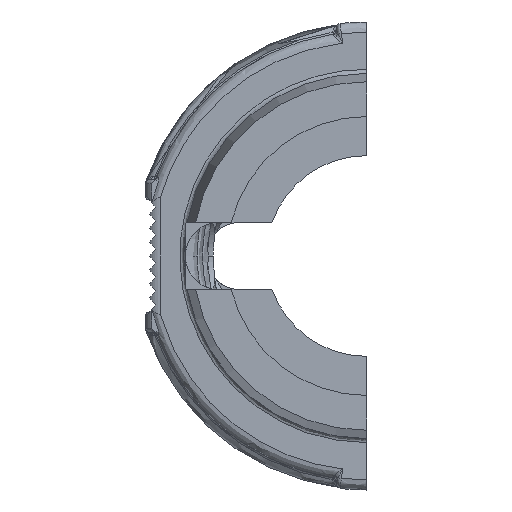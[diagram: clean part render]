
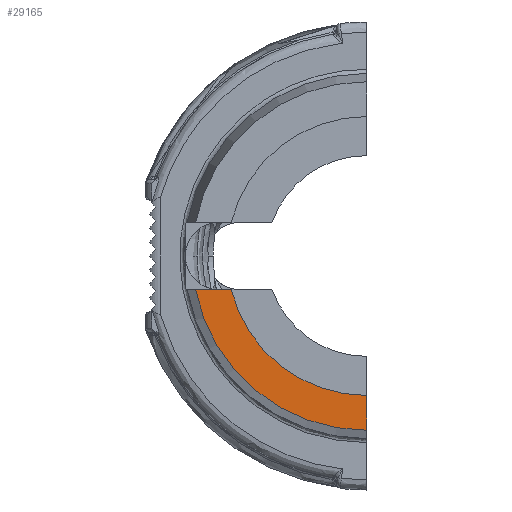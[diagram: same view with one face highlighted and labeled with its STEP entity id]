
A CAD part, left-side view. The second image highlights one B-rep face of the part: STEP entity #29165.
In plain terms, the highlighted planar face has unit normal (-1, 0, 0).
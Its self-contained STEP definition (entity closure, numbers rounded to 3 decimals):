
#5806 = DIRECTION ( 'NONE',  ( -1., 0., 0. ) ) ;
#8012 = AXIS2_PLACEMENT_3D ( 'NONE', #43436, #5806, #49741 ) ;
#8236 = CIRCLE ( 'NONE', #73202, 17.399 ) ;
#11814 = DIRECTION ( 'NONE',  ( 0., 1., 0. ) ) ;
#12703 = CARTESIAN_POINT ( 'NONE',  ( 0., 0., 0. ) ) ;
#12871 = CARTESIAN_POINT ( 'NONE',  ( 0., 0., 19.57 ) ) ;
#14411 = VECTOR ( 'NONE', #24136, 1000. ) ;
#19050 = DIRECTION ( 'NONE',  ( 0., -1., 0. ) ) ;
#19206 = DIRECTION ( 'NONE',  ( -1., 0., 0. ) ) ;
#22582 = VERTEX_POINT ( 'NONE', #62222 ) ;
#23591 = CARTESIAN_POINT ( 'NONE',  ( 0., 0., -23.818 ) ) ;
#24136 = DIRECTION ( 'NONE',  ( 0., 0., 1. ) ) ;
#24462 = CIRCLE ( 'NONE', #8012, 21.74 ) ;
#29165 = ADVANCED_FACE ( 'NONE', ( #41423 ), #50200, .T. ) ;
#30798 = VERTEX_POINT ( 'NONE', #72351 ) ;
#32179 = VECTOR ( 'NONE', #11814, 1000. ) ;
#32876 = AXIS2_PLACEMENT_3D ( 'NONE', #12871, #19206, #63117 ) ;
#36109 = ORIENTED_EDGE ( 'NONE', *, *, #81180, .T. ) ;
#37776 = ORIENTED_EDGE ( 'NONE', *, *, #70221, .T. ) ;
#41423 = FACE_OUTER_BOUND ( 'NONE', #62522, .T. ) ;
#43436 = CARTESIAN_POINT ( 'NONE',  ( 0., 0., 0. ) ) ;
#44858 = VERTEX_POINT ( 'NONE', #53710 ) ;
#45672 = ORIENTED_EDGE ( 'NONE', *, *, #50389, .T. ) ;
#49294 = CARTESIAN_POINT ( 'NONE',  ( 0., 0., -21.74 ) ) ;
#49741 = DIRECTION ( 'NONE',  ( 0., 1., 0. ) ) ;
#50200 = PLANE ( 'NONE',  #32876 ) ;
#50389 = EDGE_CURVE ( 'NONE', #44858, #22582, #8236, .T. ) ;
#53710 = CARTESIAN_POINT ( 'NONE',  ( 0., 0., -17.399 ) ) ;
#56635 = DIRECTION ( 'NONE',  ( 1., 0., 0. ) ) ;
#62222 = CARTESIAN_POINT ( 'NONE',  ( 0., 16.887, -4.191 ) ) ;
#62522 = EDGE_LOOP ( 'NONE', ( #37776, #45672, #36109, #67877 ) ) ;
#62575 = LINE ( 'NONE', #23591, #14411 ) ;
#63117 = DIRECTION ( 'NONE',  ( 0., 0., 1. ) ) ;
#66090 = EDGE_CURVE ( 'NONE', #30798, #76985, #24462, .T. ) ;
#67877 = ORIENTED_EDGE ( 'NONE', *, *, #66090, .T. ) ;
#68638 = CARTESIAN_POINT ( 'NONE',  ( 0., 0., -4.191 ) ) ;
#70221 = EDGE_CURVE ( 'NONE', #76985, #44858, #62575, .T. ) ;
#72351 = CARTESIAN_POINT ( 'NONE',  ( 0., 21.333, -4.191 ) ) ;
#73202 = AXIS2_PLACEMENT_3D ( 'NONE', #12703, #56635, #19050 ) ;
#76985 = VERTEX_POINT ( 'NONE', #49294 ) ;
#80261 = LINE ( 'NONE', #68638, #32179 ) ;
#81180 = EDGE_CURVE ( 'NONE', #22582, #30798, #80261, .T. ) ;
